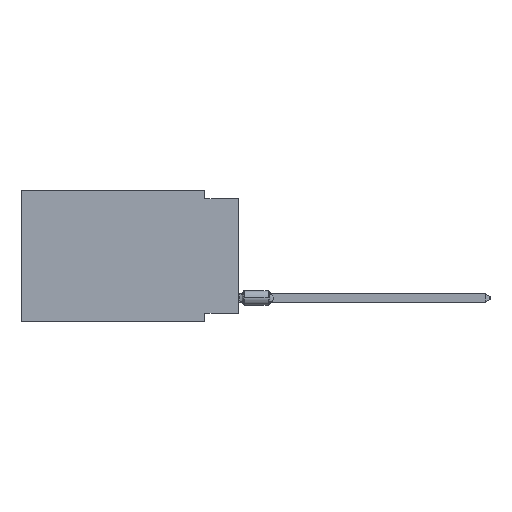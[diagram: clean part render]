
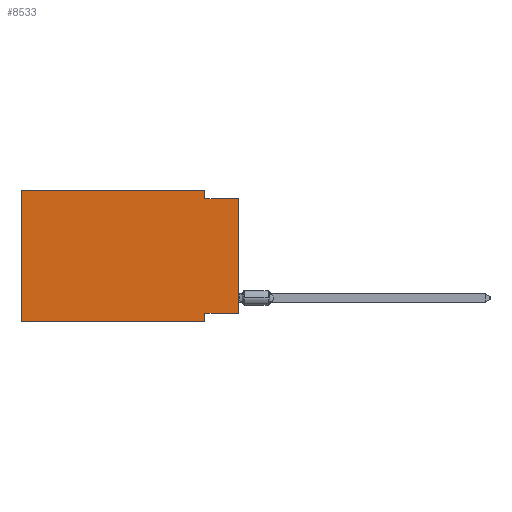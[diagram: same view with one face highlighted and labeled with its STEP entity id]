
A CAD part, left-side view. The second image highlights one B-rep face of the part: STEP entity #8533.
In plain terms, the highlighted planar face has unit normal (-1, 0, 0).
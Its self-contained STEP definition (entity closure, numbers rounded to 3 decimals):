
#469 = EDGE_CURVE ( 'NONE', #15264, #30949, #22405, .T. ) ;
#2178 = PLANE ( 'NONE',  #45687 ) ;
#2442 = DIRECTION ( 'NONE',  ( 0., 0., 1. ) ) ;
#2733 = CARTESIAN_POINT ( 'NONE',  ( 0., 0., -0.635 ) ) ;
#3285 = VECTOR ( 'NONE', #29604, 1000. ) ;
#3324 = CARTESIAN_POINT ( 'NONE',  ( 0., 0., -0.635 ) ) ;
#3693 = VECTOR ( 'NONE', #40415, 1000. ) ;
#3973 = VECTOR ( 'NONE', #28025, 1000. ) ;
#4158 = EDGE_CURVE ( 'NONE', #33739, #11126, #14559, .T. ) ;
#5458 = CARTESIAN_POINT ( 'NONE',  ( 0., 2.54, -9.906 ) ) ;
#7870 = CARTESIAN_POINT ( 'NONE',  ( 0., 0., -9.271 ) ) ;
#8366 = LINE ( 'NONE', #36569, #3285 ) ;
#8533 = ADVANCED_FACE ( 'NONE', ( #33378 ), #2178, .F. ) ;
#8765 = ORIENTED_EDGE ( 'NONE', *, *, #11639, .F. ) ;
#10258 = LINE ( 'NONE', #3324, #27415 ) ;
#10359 = EDGE_CURVE ( 'NONE', #36323, #20590, #42593, .T. ) ;
#10489 = LINE ( 'NONE', #41922, #3973 ) ;
#11126 = VERTEX_POINT ( 'NONE', #43341 ) ;
#11639 = EDGE_CURVE ( 'NONE', #36323, #33739, #43656, .T. ) ;
#12050 = ORIENTED_EDGE ( 'NONE', *, *, #34784, .F. ) ;
#12163 = CARTESIAN_POINT ( 'NONE',  ( 0., 16.383, -9.906 ) ) ;
#12998 = VECTOR ( 'NONE', #32130, 1000. ) ;
#14559 = LINE ( 'NONE', #38830, #12998 ) ;
#15264 = VERTEX_POINT ( 'NONE', #36222 ) ;
#15444 = VERTEX_POINT ( 'NONE', #17725 ) ;
#15813 = CARTESIAN_POINT ( 'NONE',  ( 0., 16.383, 0. ) ) ;
#16660 = EDGE_CURVE ( 'NONE', #11126, #15444, #8366, .T. ) ;
#17725 = CARTESIAN_POINT ( 'NONE',  ( 0., 2.54, -0.635 ) ) ;
#18094 = CARTESIAN_POINT ( 'NONE',  ( 0., 16.383, 0. ) ) ;
#18552 = CARTESIAN_POINT ( 'NONE',  ( 0., 2.54, -9.271 ) ) ;
#19371 = CARTESIAN_POINT ( 'NONE',  ( 0., 16.383, 0. ) ) ;
#19744 = CARTESIAN_POINT ( 'NONE',  ( 0., 0., 0. ) ) ;
#20115 = VECTOR ( 'NONE', #29571, 1000. ) ;
#20549 = EDGE_CURVE ( 'NONE', #15264, #42022, #23220, .T. ) ;
#20590 = VERTEX_POINT ( 'NONE', #5458 ) ;
#21625 = ORIENTED_EDGE ( 'NONE', *, *, #4158, .F. ) ;
#21770 = CARTESIAN_POINT ( 'NONE',  ( 0., 16.383, -9.906 ) ) ;
#22405 = LINE ( 'NONE', #7870, #20115 ) ;
#22561 = EDGE_CURVE ( 'NONE', #30949, #20590, #10489, .T. ) ;
#23220 = LINE ( 'NONE', #19744, #31876 ) ;
#24334 = DIRECTION ( 'NONE',  ( 0., -1., 0. ) ) ;
#25022 = ORIENTED_EDGE ( 'NONE', *, *, #16660, .F. ) ;
#25143 = ORIENTED_EDGE ( 'NONE', *, *, #10359, .T. ) ;
#26389 = ORIENTED_EDGE ( 'NONE', *, *, #20549, .T. ) ;
#27415 = VECTOR ( 'NONE', #24334, 1000. ) ;
#28001 = DIRECTION ( 'NONE',  ( 0., -1., 0. ) ) ;
#28025 = DIRECTION ( 'NONE',  ( 0., 0., -1. ) ) ;
#29571 = DIRECTION ( 'NONE',  ( 0., 1., 0. ) ) ;
#29604 = DIRECTION ( 'NONE',  ( 0., 0., -1. ) ) ;
#30124 = DIRECTION ( 'NONE',  ( 1., 0., 0. ) ) ;
#30949 = VERTEX_POINT ( 'NONE', #18552 ) ;
#31876 = VECTOR ( 'NONE', #2442, 1000. ) ;
#32130 = DIRECTION ( 'NONE',  ( 0., -1., 0. ) ) ;
#32153 = VECTOR ( 'NONE', #28001, 1000. ) ;
#32742 = ORIENTED_EDGE ( 'NONE', *, *, #22561, .F. ) ;
#33378 = FACE_OUTER_BOUND ( 'NONE', #43416, .T. ) ;
#33739 = VERTEX_POINT ( 'NONE', #18094 ) ;
#34469 = ORIENTED_EDGE ( 'NONE', *, *, #469, .F. ) ;
#34784 = EDGE_CURVE ( 'NONE', #15444, #42022, #10258, .T. ) ;
#36222 = CARTESIAN_POINT ( 'NONE',  ( 0., 0., -9.271 ) ) ;
#36323 = VERTEX_POINT ( 'NONE', #12163 ) ;
#36569 = CARTESIAN_POINT ( 'NONE',  ( 0., 2.54, 0. ) ) ;
#37307 = DIRECTION ( 'NONE',  ( 0., 0., -1. ) ) ;
#38830 = CARTESIAN_POINT ( 'NONE',  ( 0., 16.383, 0. ) ) ;
#40415 = DIRECTION ( 'NONE',  ( 0., 0., 1. ) ) ;
#41922 = CARTESIAN_POINT ( 'NONE',  ( 0., 2.54, -9.906 ) ) ;
#42022 = VERTEX_POINT ( 'NONE', #2733 ) ;
#42593 = LINE ( 'NONE', #21770, #32153 ) ;
#43341 = CARTESIAN_POINT ( 'NONE',  ( 0., 2.54, 0. ) ) ;
#43416 = EDGE_LOOP ( 'NONE', ( #26389, #12050, #25022, #21625, #8765, #25143, #32742, #34469 ) ) ;
#43656 = LINE ( 'NONE', #19371, #3693 ) ;
#45687 = AXIS2_PLACEMENT_3D ( 'NONE', #15813, #30124, #37307 ) ;
